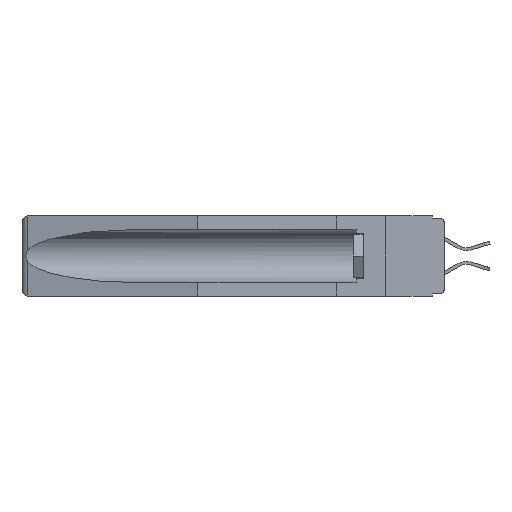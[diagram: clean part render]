
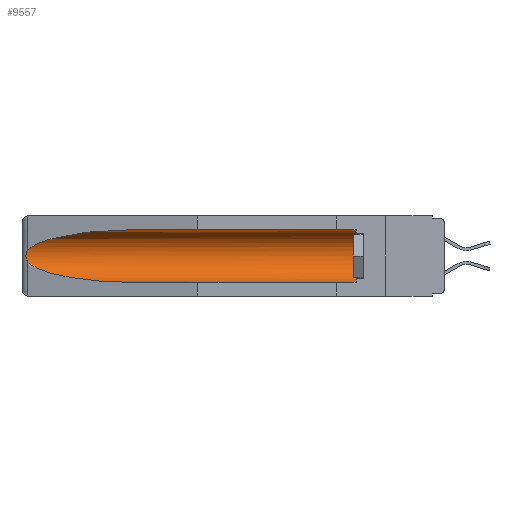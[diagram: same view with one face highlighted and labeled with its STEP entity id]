
A CAD part, left-side view. The second image highlights one B-rep face of the part: STEP entity #9557.
In plain terms, the highlighted cylindrical face has radius 2.857 mm (diameter 5.715 mm), a partial arc.
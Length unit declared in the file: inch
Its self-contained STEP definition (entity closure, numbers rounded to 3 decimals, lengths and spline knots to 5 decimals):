
#148 = CARTESIAN_POINT ( 'NONE',  ( 0.155, -0.30754, -0.284 ) ) ;
#337 = CARTESIAN_POINT ( 'NONE',  ( 0.155, -0.30754, -0.059 ) ) ;
#439 = CYLINDRICAL_SURFACE ( 'NONE', #1836, 0.1125 ) ;
#845 = B_SPLINE_CURVE_WITH_KNOTS ( 'NONE', 3,
 ( #10956, #15624, #12639, #9672, #11151, #3292, #1894, #3552, #14072, #8060 ),
 .UNSPECIFIED., .F., .F.,
 ( 4, 2, 2, 2, 4 ),
 ( 0., 0.00029, 0.00058, 0.00087, 0.00117 ),
 .UNSPECIFIED. ) ;
#1639 = ORIENTED_EDGE ( 'NONE', *, *, #4712, .T. ) ;
#1803 = DIRECTION ( 'NONE',  ( 0., 0., 1. ) ) ;
#1836 = AXIS2_PLACEMENT_3D ( 'NONE', #2063, #12613, #1803 ) ;
#1894 = CARTESIAN_POINT ( 'NONE',  ( 0.2673, 1.53269, -0.17917 ) ) ;
#1923 = AXIS2_PLACEMENT_3D ( 'NONE', #19822, #4542, #15335 ) ;
#2063 = CARTESIAN_POINT ( 'NONE',  ( 0.155, -0.30754, -0.1715 ) ) ;
#3292 = CARTESIAN_POINT ( 'NONE',  ( 0.2675, 1.53308, -0.17534 ) ) ;
#3475 = CARTESIAN_POINT ( 'NONE',  ( 0.25451, 1.48313, -0.09465 ) ) ;
#3552 = CARTESIAN_POINT ( 'NONE',  ( 0.26655, 1.53094, -0.18657 ) ) ;
#3675 = CARTESIAN_POINT ( 'NONE',  ( 0.155, 1.07973, -0.059 ) ) ;
#3990 = EDGE_CURVE ( 'NONE', #7244, #4897, #845, .T. ) ;
#4100 = VECTOR ( 'NONE', #9600, 39.37008 ) ;
#4542 = DIRECTION ( 'NONE',  ( 0., -1., 0. ) ) ;
#4712 = EDGE_CURVE ( 'NONE', #4897, #5820, #18495, .T. ) ;
#4751 = FACE_OUTER_BOUND ( 'NONE', #19877, .T. ) ;
#4897 = VERTEX_POINT ( 'NONE', #12329 ) ;
#4950 = CARTESIAN_POINT ( 'NONE',  ( 0.26537, 1.52718, -0.14972 ) ) ;
#5086 = ORIENTED_EDGE ( 'NONE', *, *, #7082, .T. ) ;
#5224 = ORIENTED_EDGE ( 'NONE', *, *, #13725, .F. ) ;
#5281 = CARTESIAN_POINT ( 'NONE',  ( 0.26537, 1.52718, -0.14972 ) ) ;
#5820 = VERTEX_POINT ( 'NONE', #19275 ) ;
#5928 = CARTESIAN_POINT ( 'NONE',  ( 0.26537, 1.52718, -0.19328 ) ) ;
#7082 = EDGE_CURVE ( 'NONE', #16498, #15527, #9408, .T. ) ;
#7244 = VERTEX_POINT ( 'NONE', #5281 ) ;
#7532 = EDGE_CURVE ( 'NONE', #12178, #16498, #16637, .T. ) ;
#7797 = ORIENTED_EDGE ( 'NONE', *, *, #11830, .T. ) ;
#8060 = CARTESIAN_POINT ( 'NONE',  ( 0.26537, 1.52718, -0.19328 ) ) ;
#8968 = CARTESIAN_POINT ( 'NONE',  ( 0.155, 1.07973, -0.284 ) ) ;
#9408 = LINE ( 'NONE', #337, #4100 ) ;
#9557 = ADVANCED_FACE ( 'NONE', ( #4751 ), #439, .F. ) ;
#9600 = DIRECTION ( 'NONE',  ( 0., 1., 0. ) ) ;
#9672 = CARTESIAN_POINT ( 'NONE',  ( 0.2673, 1.5327, -0.16383 ) ) ;
#10956 = CARTESIAN_POINT ( 'NONE',  ( 0.26537, 1.52718, -0.14972 ) ) ;
#11151 = CARTESIAN_POINT ( 'NONE',  ( 0.2675, 1.53308, -0.16763 ) ) ;
#11830 = EDGE_CURVE ( 'NONE', #15527, #7244, #16655, .T. ) ;
#12097 = CARTESIAN_POINT ( 'NONE',  ( 0.21114, 1.30732, -0.059 ) ) ;
#12178 = VERTEX_POINT ( 'NONE', #17706 ) ;
#12231 = CARTESIAN_POINT ( 'NONE',  ( 0.155, 1.07973, -0.059 ) ) ;
#12329 = CARTESIAN_POINT ( 'NONE',  ( 0.26537, 1.52718, -0.19328 ) ) ;
#12613 = DIRECTION ( 'NONE',  ( 0., 1., 0. ) ) ;
#12639 = CARTESIAN_POINT ( 'NONE',  ( 0.26654, 1.53092, -0.15636 ) ) ;
#12688 = VECTOR ( 'NONE', #15642, 39.37008 ) ;
#13422 = LINE ( 'NONE', #148, #12688 ) ;
#13725 = EDGE_CURVE ( 'NONE', #12178, #5820, #13422, .T. ) ;
#14072 = CARTESIAN_POINT ( 'NONE',  ( 0.26597, 1.5296, -0.19026 ) ) ;
#15026 = ORIENTED_EDGE ( 'NONE', *, *, #7532, .T. ) ;
#15335 = DIRECTION ( 'NONE',  ( 0., 0., 1. ) ) ;
#15527 = VERTEX_POINT ( 'NONE', #3675 ) ;
#15624 = CARTESIAN_POINT ( 'NONE',  ( 0.26597, 1.52961, -0.15275 ) ) ;
#15642 = DIRECTION ( 'NONE',  ( 0., 1., 0. ) ) ;
#16498 = VERTEX_POINT ( 'NONE', #19455 ) ;
#16637 = CIRCLE ( 'NONE', #1923, 0.1125 ) ;
#16655 =( BOUNDED_CURVE ( )  B_SPLINE_CURVE ( 3, ( #12231, #12097, #3475, #4950 ),
 .UNSPECIFIED., .F., .F. ) 
 B_SPLINE_CURVE_WITH_KNOTS ( ( 4, 4 ),
 ( 4.71239, 6.08839 ),
 .UNSPECIFIED. ) 
 CURVE ( )  GEOMETRIC_REPRESENTATION_ITEM ( )  RATIONAL_B_SPLINE_CURVE ( ( 1., 0.848, 0.848, 1. ) ) 
 REPRESENTATION_ITEM ( '' )  );
#17706 = CARTESIAN_POINT ( 'NONE',  ( 0.155, 0.126, -0.284 ) ) ;
#18151 = CARTESIAN_POINT ( 'NONE',  ( 0.25451, 1.48313, -0.24835 ) ) ;
#18284 = CARTESIAN_POINT ( 'NONE',  ( 0.21114, 1.30732, -0.284 ) ) ;
#18495 =( BOUNDED_CURVE ( )  B_SPLINE_CURVE ( 3, ( #5928, #18151, #18284, #8968 ),
 .UNSPECIFIED., .F., .F. ) 
 B_SPLINE_CURVE_WITH_KNOTS ( ( 4, 4 ),
 ( 0.1948, 1.5708 ),
 .UNSPECIFIED. ) 
 CURVE ( )  GEOMETRIC_REPRESENTATION_ITEM ( )  RATIONAL_B_SPLINE_CURVE ( ( 1., 0.848, 0.848, 1. ) ) 
 REPRESENTATION_ITEM ( '' )  );
#19270 = ORIENTED_EDGE ( 'NONE', *, *, #3990, .T. ) ;
#19275 = CARTESIAN_POINT ( 'NONE',  ( 0.155, 1.07973, -0.284 ) ) ;
#19455 = CARTESIAN_POINT ( 'NONE',  ( 0.155, 0.126, -0.059 ) ) ;
#19822 = CARTESIAN_POINT ( 'NONE',  ( 0.155, 0.126, -0.1715 ) ) ;
#19877 = EDGE_LOOP ( 'NONE', ( #7797, #19270, #1639, #5224, #15026, #5086 ) ) ;
